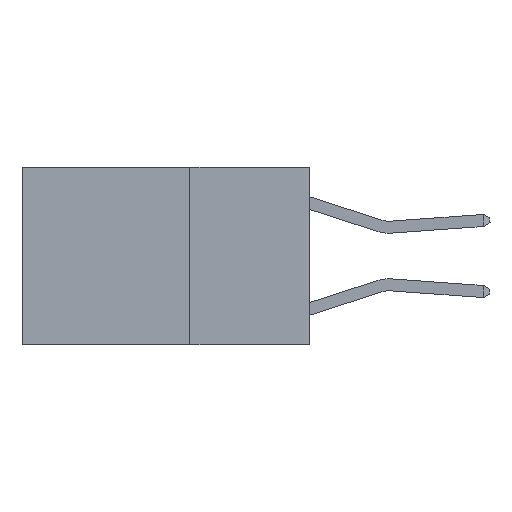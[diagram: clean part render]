
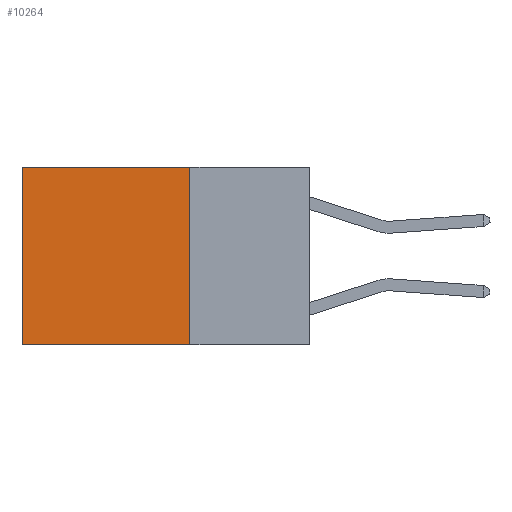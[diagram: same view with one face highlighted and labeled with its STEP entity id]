
A CAD part, left-side view. The second image highlights one B-rep face of the part: STEP entity #10264.
In plain terms, the highlighted planar face has unit normal (-1, 0, 0).
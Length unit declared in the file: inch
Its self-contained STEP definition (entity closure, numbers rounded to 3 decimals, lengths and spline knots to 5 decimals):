
#2825 = FACE_OUTER_BOUND ( 'NONE', #29111, .T. ) ;
#3449 = CARTESIAN_POINT ( 'NONE',  ( 0.2625, 0.6, -0.37 ) ) ;
#4384 = DIRECTION ( 'NONE',  ( 1., 0., 0. ) ) ;
#4415 = EDGE_CURVE ( 'NONE', #11764, #13210, #25948, .T. ) ;
#5094 = ORIENTED_EDGE ( 'NONE', *, *, #10303, .F. ) ;
#5162 = VECTOR ( 'NONE', #9272, 39.37008 ) ;
#6289 = LINE ( 'NONE', #16454, #11499 ) ;
#6305 = EDGE_CURVE ( 'NONE', #13210, #13433, #31331, .T. ) ;
#6658 = ORIENTED_EDGE ( 'NONE', *, *, #20007, .F. ) ;
#8461 = DIRECTION ( 'NONE',  ( 0., 0., -1. ) ) ;
#8572 = VERTEX_POINT ( 'NONE', #8888 ) ;
#8888 = CARTESIAN_POINT ( 'NONE',  ( 0.2625, 0.25, -0.37 ) ) ;
#9204 = CARTESIAN_POINT ( 'NONE',  ( 0.2625, 0.25, 0. ) ) ;
#9272 = DIRECTION ( 'NONE',  ( 0., 0., -1. ) ) ;
#9783 = DIRECTION ( 'NONE',  ( 0., 1., 0. ) ) ;
#10264 = ADVANCED_FACE ( 'NONE', ( #2825 ), #27769, .F. ) ;
#10303 = EDGE_CURVE ( 'NONE', #11764, #8572, #25540, .T. ) ;
#11499 = VECTOR ( 'NONE', #9783, 39.37008 ) ;
#11764 = VERTEX_POINT ( 'NONE', #16685 ) ;
#13210 = VERTEX_POINT ( 'NONE', #16691 ) ;
#13433 = VERTEX_POINT ( 'NONE', #3449 ) ;
#13576 = CARTESIAN_POINT ( 'NONE',  ( 0.2625, 0.25, 0. ) ) ;
#16454 = CARTESIAN_POINT ( 'NONE',  ( 0.2625, 0.25, -0.37 ) ) ;
#16652 = AXIS2_PLACEMENT_3D ( 'NONE', #21447, #4384, #8461 ) ;
#16685 = CARTESIAN_POINT ( 'NONE',  ( 0.2625, 0.25, 0. ) ) ;
#16691 = CARTESIAN_POINT ( 'NONE',  ( 0.2625, 0.6, 0. ) ) ;
#20007 = EDGE_CURVE ( 'NONE', #8572, #13433, #6289, .T. ) ;
#20742 = VECTOR ( 'NONE', #23262, 39.37008 ) ;
#21447 = CARTESIAN_POINT ( 'NONE',  ( 0.2625, 0.25, 0. ) ) ;
#23262 = DIRECTION ( 'NONE',  ( 0., 0., -1. ) ) ;
#23365 = DIRECTION ( 'NONE',  ( 0., 1., 0. ) ) ;
#25540 = LINE ( 'NONE', #9204, #20742 ) ;
#25948 = LINE ( 'NONE', #13576, #26733 ) ;
#26369 = ORIENTED_EDGE ( 'NONE', *, *, #4415, .T. ) ;
#26733 = VECTOR ( 'NONE', #23365, 39.37008 ) ;
#27769 = PLANE ( 'NONE',  #16652 ) ;
#28751 = CARTESIAN_POINT ( 'NONE',  ( 0.2625, 0.6, 0. ) ) ;
#29111 = EDGE_LOOP ( 'NONE', ( #29193, #6658, #5094, #26369 ) ) ;
#29193 = ORIENTED_EDGE ( 'NONE', *, *, #6305, .T. ) ;
#31331 = LINE ( 'NONE', #28751, #5162 ) ;
